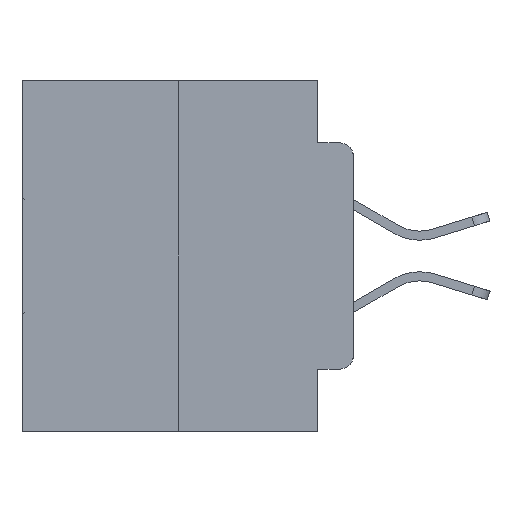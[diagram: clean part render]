
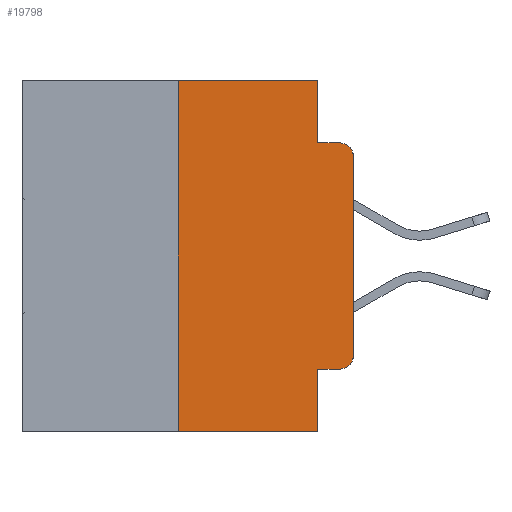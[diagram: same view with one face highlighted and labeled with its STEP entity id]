
A CAD part, left-side view. The second image highlights one B-rep face of the part: STEP entity #19798.
In plain terms, the highlighted planar face has unit normal (-1, 0, 0).
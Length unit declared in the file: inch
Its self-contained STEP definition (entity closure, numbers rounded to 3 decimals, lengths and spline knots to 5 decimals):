
#496 = VECTOR ( 'NONE', #19119, 39.37008 ) ;
#547 = CARTESIAN_POINT ( 'NONE',  ( 0., 0., 0. ) ) ;
#796 = VERTEX_POINT ( 'NONE', #11073 ) ;
#1144 = VECTOR ( 'NONE', #21745, 39.37008 ) ;
#1560 = CARTESIAN_POINT ( 'NONE',  ( 0., 0.25, -0.5 ) ) ;
#1665 = VECTOR ( 'NONE', #11184, 39.37008 ) ;
#2151 = EDGE_CURVE ( 'NONE', #19559, #796, #14776, .T. ) ;
#2266 = EDGE_LOOP ( 'NONE', ( #16659, #11967, #21793, #15180, #13323, #2960, #5273, #15784, #21711, #13125 ) ) ;
#2834 = DIRECTION ( 'NONE',  ( -1., 0., 0. ) ) ;
#2914 = EDGE_CURVE ( 'NONE', #796, #5096, #8687, .T. ) ;
#2960 = ORIENTED_EDGE ( 'NONE', *, *, #26638, .F. ) ;
#3550 = CARTESIAN_POINT ( 'NONE',  ( 0., 0.02, -0.3915 ) ) ;
#4149 = LINE ( 'NONE', #4296, #22126 ) ;
#4282 = CARTESIAN_POINT ( 'NONE',  ( 0., 0.051, -0.4115 ) ) ;
#4296 = CARTESIAN_POINT ( 'NONE',  ( 0., 0.25, 0. ) ) ;
#5096 = VERTEX_POINT ( 'NONE', #7109 ) ;
#5273 = ORIENTED_EDGE ( 'NONE', *, *, #20409, .T. ) ;
#5994 = DIRECTION ( 'NONE',  ( -1., 0., 0. ) ) ;
#6085 = CARTESIAN_POINT ( 'NONE',  ( 0., 0.051, -0.0885 ) ) ;
#6619 = EDGE_CURVE ( 'NONE', #9869, #5096, #14058, .T. ) ;
#7109 = CARTESIAN_POINT ( 'NONE',  ( 0., 0.02, -0.0885 ) ) ;
#7844 = VERTEX_POINT ( 'NONE', #1560 ) ;
#8144 = VERTEX_POINT ( 'NONE', #19892 ) ;
#8687 = CIRCLE ( 'NONE', #28215, 0.02 ) ;
#8756 = CARTESIAN_POINT ( 'NONE',  ( 0., 0.473, 0. ) ) ;
#8768 = CARTESIAN_POINT ( 'NONE',  ( 0., 0.02, -0.4115 ) ) ;
#9655 = CARTESIAN_POINT ( 'NONE',  ( 0., 0.051, -0.5 ) ) ;
#9869 = VERTEX_POINT ( 'NONE', #6085 ) ;
#10761 = PLANE ( 'NONE',  #14297 ) ;
#10921 = EDGE_CURVE ( 'NONE', #29100, #19559, #30154, .T. ) ;
#11073 = CARTESIAN_POINT ( 'NONE',  ( 0., 0., -0.1085 ) ) ;
#11184 = DIRECTION ( 'NONE',  ( 0., -1., 0. ) ) ;
#11612 = DIRECTION ( 'NONE',  ( 0., -1., 0. ) ) ;
#11664 = VERTEX_POINT ( 'NONE', #18310 ) ;
#11732 = CARTESIAN_POINT ( 'NONE',  ( 0., 0.051, 0. ) ) ;
#11736 = CARTESIAN_POINT ( 'NONE',  ( 0., 0.02, -0.1085 ) ) ;
#11967 = ORIENTED_EDGE ( 'NONE', *, *, #2914, .T. ) ;
#12077 = CARTESIAN_POINT ( 'NONE',  ( 0., 0.051, -0.0885 ) ) ;
#12414 = VECTOR ( 'NONE', #15000, 39.37008 ) ;
#12458 = DIRECTION ( 'NONE',  ( 0., 0., 1. ) ) ;
#13125 = ORIENTED_EDGE ( 'NONE', *, *, #10921, .T. ) ;
#13323 = ORIENTED_EDGE ( 'NONE', *, *, #29524, .F. ) ;
#13507 = DIRECTION ( 'NONE',  ( 0., 0., -1. ) ) ;
#13680 = VERTEX_POINT ( 'NONE', #9655 ) ;
#14058 = LINE ( 'NONE', #12077, #496 ) ;
#14297 = AXIS2_PLACEMENT_3D ( 'NONE', #8756, #29572, #13507 ) ;
#14776 = LINE ( 'NONE', #547, #29648 ) ;
#15000 = DIRECTION ( 'NONE',  ( 0., 0., -1. ) ) ;
#15180 = ORIENTED_EDGE ( 'NONE', *, *, #27933, .F. ) ;
#15784 = ORIENTED_EDGE ( 'NONE', *, *, #23338, .F. ) ;
#16659 = ORIENTED_EDGE ( 'NONE', *, *, #2151, .T. ) ;
#16978 = AXIS2_PLACEMENT_3D ( 'NONE', #3550, #5994, #17034 ) ;
#16986 = LINE ( 'NONE', #18984, #1144 ) ;
#17034 = DIRECTION ( 'NONE',  ( 0., 0., -1. ) ) ;
#17908 = DIRECTION ( 'NONE',  ( 0., 0., 1. ) ) ;
#18310 = CARTESIAN_POINT ( 'NONE',  ( 0., 0.25, 0. ) ) ;
#18342 = LINE ( 'NONE', #24953, #26585 ) ;
#18984 = CARTESIAN_POINT ( 'NONE',  ( 0., 0.051, 0. ) ) ;
#19119 = DIRECTION ( 'NONE',  ( 0., -1., 0. ) ) ;
#19559 = VERTEX_POINT ( 'NONE', #21200 ) ;
#19798 = ADVANCED_FACE ( 'NONE', ( #20245 ), #10761, .F. ) ;
#19892 = CARTESIAN_POINT ( 'NONE',  ( 0., 0.051, -0.4115 ) ) ;
#20194 = CARTESIAN_POINT ( 'NONE',  ( 0., 0.051, 0. ) ) ;
#20245 = FACE_OUTER_BOUND ( 'NONE', #2266, .T. ) ;
#20409 = EDGE_CURVE ( 'NONE', #7844, #13680, #30136, .T. ) ;
#21200 = CARTESIAN_POINT ( 'NONE',  ( 0., 0., -0.3915 ) ) ;
#21711 = ORIENTED_EDGE ( 'NONE', *, *, #23526, .T. ) ;
#21745 = DIRECTION ( 'NONE',  ( 0., 0., -1. ) ) ;
#21793 = ORIENTED_EDGE ( 'NONE', *, *, #6619, .F. ) ;
#22126 = VECTOR ( 'NONE', #17908, 39.37008 ) ;
#22975 = LINE ( 'NONE', #4282, #1665 ) ;
#23338 = EDGE_CURVE ( 'NONE', #8144, #13680, #29668, .T. ) ;
#23526 = EDGE_CURVE ( 'NONE', #8144, #29100, #22975, .T. ) ;
#24953 = CARTESIAN_POINT ( 'NONE',  ( 0., 0.473, 0. ) ) ;
#25560 = VECTOR ( 'NONE', #29982, 39.37008 ) ;
#25806 = DIRECTION ( 'NONE',  ( 0., 0., -1. ) ) ;
#26585 = VECTOR ( 'NONE', #11612, 39.37008 ) ;
#26638 = EDGE_CURVE ( 'NONE', #7844, #11664, #4149, .T. ) ;
#27838 = CARTESIAN_POINT ( 'NONE',  ( 0., 0.473, -0.5 ) ) ;
#27933 = EDGE_CURVE ( 'NONE', #30186, #9869, #16986, .T. ) ;
#28215 = AXIS2_PLACEMENT_3D ( 'NONE', #11736, #2834, #25806 ) ;
#29100 = VERTEX_POINT ( 'NONE', #8768 ) ;
#29524 = EDGE_CURVE ( 'NONE', #11664, #30186, #18342, .T. ) ;
#29572 = DIRECTION ( 'NONE',  ( 1., 0., 0. ) ) ;
#29648 = VECTOR ( 'NONE', #12458, 39.37008 ) ;
#29668 = LINE ( 'NONE', #20194, #12414 ) ;
#29982 = DIRECTION ( 'NONE',  ( 0., -1., 0. ) ) ;
#30136 = LINE ( 'NONE', #27838, #25560 ) ;
#30154 = CIRCLE ( 'NONE', #16978, 0.02 ) ;
#30186 = VERTEX_POINT ( 'NONE', #11732 ) ;
